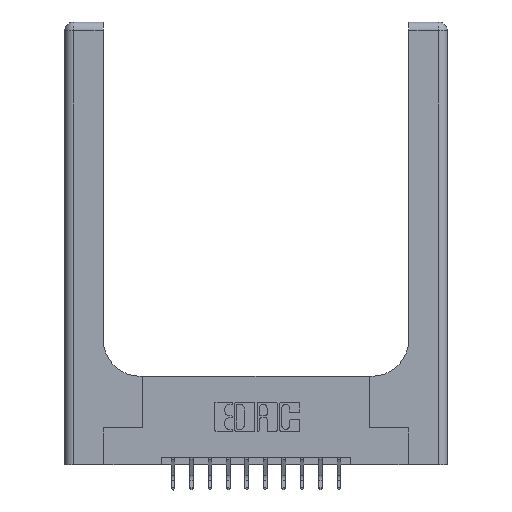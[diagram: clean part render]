
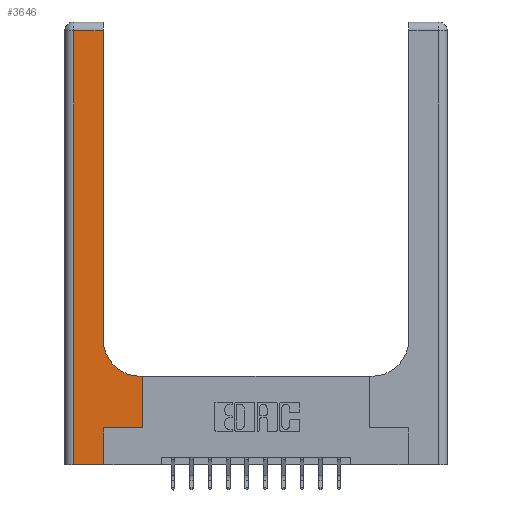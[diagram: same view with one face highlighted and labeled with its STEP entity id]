
A CAD part, top view. The second image highlights one B-rep face of the part: STEP entity #3646.
In plain terms, the highlighted planar face has unit normal (0, 0, 1).
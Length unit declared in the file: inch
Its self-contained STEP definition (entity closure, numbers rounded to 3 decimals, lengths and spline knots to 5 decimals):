
#306 = DIRECTION ( 'NONE',  ( 1., 0., 0. ) ) ;
#324 = VECTOR ( 'NONE', #601, 39.37008 ) ;
#601 = DIRECTION ( 'NONE',  ( 0., 1., 0. ) ) ;
#663 = EDGE_CURVE ( 'NONE', #3128, #12444, #4853, .T. ) ;
#770 = VECTOR ( 'NONE', #3097, 39.37008 ) ;
#780 = VECTOR ( 'NONE', #6343, 39.37008 ) ;
#1179 = CARTESIAN_POINT ( 'NONE',  ( 0.528, 0.25, 0.37 ) ) ;
#1345 = EDGE_CURVE ( 'NONE', #7029, #3024, #3852, .T. ) ;
#1531 = VECTOR ( 'NONE', #14944, 39.37008 ) ;
#2264 = EDGE_CURVE ( 'NONE', #8607, #3128, #9928, .T. ) ;
#2374 = VERTEX_POINT ( 'NONE', #4581 ) ;
#2529 = AXIS2_PLACEMENT_3D ( 'NONE', #3514, #7334, #16095 ) ;
#3013 = CARTESIAN_POINT ( 'NONE',  ( 0.265, 0.25, 0.37 ) ) ;
#3024 = VERTEX_POINT ( 'NONE', #3013 ) ;
#3097 = DIRECTION ( 'NONE',  ( 0., 1., 0. ) ) ;
#3128 = VERTEX_POINT ( 'NONE', #5888 ) ;
#3139 = VECTOR ( 'NONE', #11129, 39.37008 ) ;
#3264 = ORIENTED_EDGE ( 'NONE', *, *, #4019, .T. ) ;
#3313 = EDGE_CURVE ( 'NONE', #13005, #12976, #6944, .T. ) ;
#3514 = CARTESIAN_POINT ( 'NONE',  ( 0., 3., 0.37 ) ) ;
#3646 = ADVANCED_FACE ( 'NONE', ( #15107 ), #14815, .F. ) ;
#3670 = ORIENTED_EDGE ( 'NONE', *, *, #3313, .T. ) ;
#3852 = LINE ( 'NONE', #8201, #324 ) ;
#4019 = EDGE_CURVE ( 'NONE', #3024, #13005, #6171, .T. ) ;
#4086 = CARTESIAN_POINT ( 'NONE',  ( 0.06, 2.94, 0.37 ) ) ;
#4112 = EDGE_CURVE ( 'NONE', #2374, #7029, #11971, .T. ) ;
#4577 = ORIENTED_EDGE ( 'NONE', *, *, #4112, .T. ) ;
#4581 = CARTESIAN_POINT ( 'NONE',  ( 0.06, 0., 0.37 ) ) ;
#4728 = VERTEX_POINT ( 'NONE', #8380 ) ;
#4853 = LINE ( 'NONE', #10921, #1531 ) ;
#4896 = VECTOR ( 'NONE', #306, 39.37008 ) ;
#4976 = CARTESIAN_POINT ( 'NONE',  ( 0.26, 0.6, 0.37 ) ) ;
#5355 = CARTESIAN_POINT ( 'NONE',  ( 0.06, 3., 0.37 ) ) ;
#5562 = CARTESIAN_POINT ( 'NONE',  ( 0.26, 3., 0.37 ) ) ;
#5676 = ORIENTED_EDGE ( 'NONE', *, *, #11219, .T. ) ;
#5716 = CIRCLE ( 'NONE', #11340, 0.25 ) ;
#5888 = CARTESIAN_POINT ( 'NONE',  ( 0.26, 2.94, 0.37 ) ) ;
#6171 = LINE ( 'NONE', #13808, #780 ) ;
#6206 = DIRECTION ( 'NONE',  ( 0., 0., -1. ) ) ;
#6343 = DIRECTION ( 'NONE',  ( 1., 0., 0. ) ) ;
#6944 = LINE ( 'NONE', #15174, #770 ) ;
#7029 = VERTEX_POINT ( 'NONE', #16105 ) ;
#7334 = DIRECTION ( 'NONE',  ( 0., 0., -1. ) ) ;
#7937 = VECTOR ( 'NONE', #9218, 39.37008 ) ;
#8201 = CARTESIAN_POINT ( 'NONE',  ( 0.265, 0., 0.37 ) ) ;
#8380 = CARTESIAN_POINT ( 'NONE',  ( 0.51, 0.6, 0.37 ) ) ;
#8453 = CARTESIAN_POINT ( 'NONE',  ( 0.26, 0.85, 0.37 ) ) ;
#8596 = ORIENTED_EDGE ( 'NONE', *, *, #10085, .T. ) ;
#8607 = VERTEX_POINT ( 'NONE', #8453 ) ;
#9218 = DIRECTION ( 'NONE',  ( 0., -1., 0. ) ) ;
#9544 = ORIENTED_EDGE ( 'NONE', *, *, #1345, .T. ) ;
#9549 = ORIENTED_EDGE ( 'NONE', *, *, #16121, .T. ) ;
#9574 = DIRECTION ( 'NONE',  ( 0., 1., 0. ) ) ;
#9755 = ORIENTED_EDGE ( 'NONE', *, *, #2264, .T. ) ;
#9928 = LINE ( 'NONE', #5562, #15993 ) ;
#10085 = EDGE_CURVE ( 'NONE', #12976, #4728, #12986, .T. ) ;
#10921 = CARTESIAN_POINT ( 'NONE',  ( 0., 2.94, 0.37 ) ) ;
#11050 = CARTESIAN_POINT ( 'NONE',  ( 0.51, 0.85, 0.37 ) ) ;
#11129 = DIRECTION ( 'NONE',  ( -1., 0., 0. ) ) ;
#11219 = EDGE_CURVE ( 'NONE', #4728, #8607, #5716, .T. ) ;
#11340 = AXIS2_PLACEMENT_3D ( 'NONE', #11050, #6206, #12306 ) ;
#11971 = LINE ( 'NONE', #14064, #4896 ) ;
#12239 = ORIENTED_EDGE ( 'NONE', *, *, #663, .T. ) ;
#12306 = DIRECTION ( 'NONE',  ( 1., 0., 0. ) ) ;
#12444 = VERTEX_POINT ( 'NONE', #4086 ) ;
#12976 = VERTEX_POINT ( 'NONE', #13898 ) ;
#12986 = LINE ( 'NONE', #4976, #3139 ) ;
#13005 = VERTEX_POINT ( 'NONE', #1179 ) ;
#13808 = CARTESIAN_POINT ( 'NONE',  ( 0.265, 0.25, 0.37 ) ) ;
#13898 = CARTESIAN_POINT ( 'NONE',  ( 0.528, 0.6, 0.37 ) ) ;
#14064 = CARTESIAN_POINT ( 'NONE',  ( 0., 0., 0.37 ) ) ;
#14153 = EDGE_LOOP ( 'NONE', ( #9755, #12239, #9549, #4577, #9544, #3264, #3670, #8596, #5676 ) ) ;
#14194 = LINE ( 'NONE', #5355, #7937 ) ;
#14815 = PLANE ( 'NONE',  #2529 ) ;
#14944 = DIRECTION ( 'NONE',  ( -1., 0., 0. ) ) ;
#15107 = FACE_OUTER_BOUND ( 'NONE', #14153, .T. ) ;
#15174 = CARTESIAN_POINT ( 'NONE',  ( 0.528, 0.25, 0.37 ) ) ;
#15993 = VECTOR ( 'NONE', #9574, 39.37008 ) ;
#16095 = DIRECTION ( 'NONE',  ( -1., 0., 0. ) ) ;
#16105 = CARTESIAN_POINT ( 'NONE',  ( 0.265, 0., 0.37 ) ) ;
#16121 = EDGE_CURVE ( 'NONE', #12444, #2374, #14194, .T. ) ;
